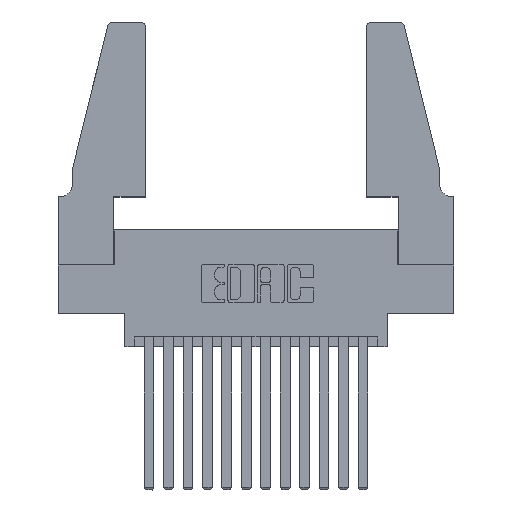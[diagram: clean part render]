
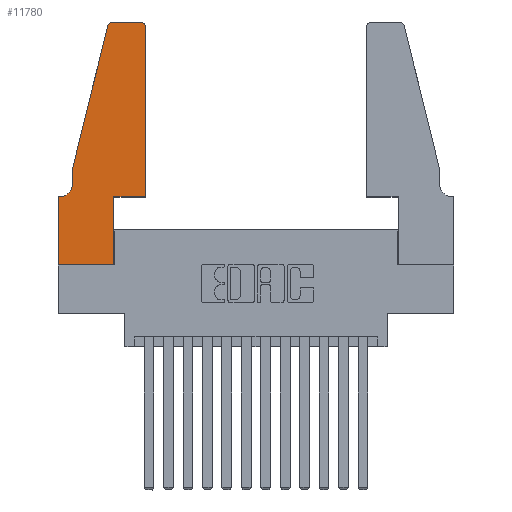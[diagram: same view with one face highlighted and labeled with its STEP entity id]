
A CAD part, top view. The second image highlights one B-rep face of the part: STEP entity #11780.
In plain terms, the highlighted planar face has unit normal (0, 0, 1).
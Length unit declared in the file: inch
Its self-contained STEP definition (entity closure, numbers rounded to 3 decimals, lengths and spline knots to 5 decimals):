
#50 = EDGE_CURVE ( 'NONE', #7303, #5042, #13932, .T. ) ;
#340 = DIRECTION ( 'NONE',  ( -0.239, -0.971, 0. ) ) ;
#411 = LINE ( 'NONE', #6189, #12069 ) ;
#577 = DIRECTION ( 'NONE',  ( 1., 0., 0. ) ) ;
#581 = CARTESIAN_POINT ( 'NONE',  ( 0., 0., 0.37 ) ) ;
#876 = CARTESIAN_POINT ( 'NONE',  ( 0.0055, 0.42, 0.37 ) ) ;
#1101 = CARTESIAN_POINT ( 'NONE',  ( 0.2865, 0., 0.37 ) ) ;
#1343 = ORIENTED_EDGE ( 'NONE', *, *, #13371, .T. ) ;
#1584 = CARTESIAN_POINT ( 'NONE',  ( 0.4205, 1.25, 0.37 ) ) ;
#1588 = DIRECTION ( 'NONE',  ( 0., 0., 1. ) ) ;
#1803 = CARTESIAN_POINT ( 'NONE',  ( 0.284, 1.22, 0.37 ) ) ;
#1908 = ORIENTED_EDGE ( 'NONE', *, *, #12167, .T. ) ;
#1970 = DIRECTION ( 'NONE',  ( 1., 0., 0. ) ) ;
#1988 = VERTEX_POINT ( 'NONE', #4067 ) ;
#2097 = VERTEX_POINT ( 'NONE', #13837 ) ;
#2110 = DIRECTION ( 'NONE',  ( 0., 0., -1. ) ) ;
#2118 = DIRECTION ( 'NONE',  ( 0., 1., 0. ) ) ;
#2516 = EDGE_CURVE ( 'NONE', #4257, #2097, #8026, .T. ) ;
#2548 = LINE ( 'NONE', #3177, #3809 ) ;
#2707 = VERTEX_POINT ( 'NONE', #11678 ) ;
#2776 = VECTOR ( 'NONE', #14270, 39.37008 ) ;
#2869 = VERTEX_POINT ( 'NONE', #1584 ) ;
#2880 = FACE_OUTER_BOUND ( 'NONE', #12619, .T. ) ;
#2902 = CARTESIAN_POINT ( 'NONE',  ( 0.4505, 0.35, 0.37 ) ) ;
#2933 = AXIS2_PLACEMENT_3D ( 'NONE', #1803, #6779, #1970 ) ;
#3019 = AXIS2_PLACEMENT_3D ( 'NONE', #876, #2110, #5719 ) ;
#3177 = CARTESIAN_POINT ( 'NONE',  ( 0.0755, 0.5, 0.37 ) ) ;
#3406 = VECTOR ( 'NONE', #7748, 39.37008 ) ;
#3809 = VECTOR ( 'NONE', #15198, 39.37008 ) ;
#4067 = CARTESIAN_POINT ( 'NONE',  ( 0.4505, 0.35, 0.37 ) ) ;
#4119 = LINE ( 'NONE', #10100, #3406 ) ;
#4257 = VERTEX_POINT ( 'NONE', #1101 ) ;
#5042 = VERTEX_POINT ( 'NONE', #15515 ) ;
#5075 = VERTEX_POINT ( 'NONE', #10425 ) ;
#5323 = CARTESIAN_POINT ( 'NONE',  ( 0.2605, 1.25, 0.37 ) ) ;
#5719 = DIRECTION ( 'NONE',  ( -1., 0., 0. ) ) ;
#5789 = VECTOR ( 'NONE', #11510, 39.37008 ) ;
#6189 = CARTESIAN_POINT ( 'NONE',  ( 0.0755, 0.35, 0.37 ) ) ;
#6210 = LINE ( 'NONE', #12662, #7722 ) ;
#6779 = DIRECTION ( 'NONE',  ( 0., 0., 1. ) ) ;
#7237 = EDGE_CURVE ( 'NONE', #13551, #9229, #15389, .T. ) ;
#7271 = CARTESIAN_POINT ( 'NONE',  ( 0.0755, 0.42, 0.37 ) ) ;
#7303 = VERTEX_POINT ( 'NONE', #12713 ) ;
#7722 = VECTOR ( 'NONE', #577, 39.37008 ) ;
#7748 = DIRECTION ( 'NONE',  ( 1., 0., 0. ) ) ;
#7757 = ORIENTED_EDGE ( 'NONE', *, *, #50, .T. ) ;
#8026 = LINE ( 'NONE', #11632, #2776 ) ;
#8221 = DIRECTION ( 'NONE',  ( 1., 0., 0. ) ) ;
#8367 = VECTOR ( 'NONE', #10159, 39.37008 ) ;
#8490 = ORIENTED_EDGE ( 'NONE', *, *, #10741, .T. ) ;
#8747 = DIRECTION ( 'NONE',  ( 1., 0., 0. ) ) ;
#8868 = CIRCLE ( 'NONE', #9159, 0.03 ) ;
#9159 = AXIS2_PLACEMENT_3D ( 'NONE', #10366, #12994, #8221 ) ;
#9229 = VERTEX_POINT ( 'NONE', #15496 ) ;
#9512 = LINE ( 'NONE', #5323, #8367 ) ;
#9833 = DIRECTION ( 'NONE',  ( -1., 0., 0. ) ) ;
#9992 = CARTESIAN_POINT ( 'NONE',  ( 0., 0.35, 0.37 ) ) ;
#10038 = AXIS2_PLACEMENT_3D ( 'NONE', #9992, #1588, #8747 ) ;
#10100 = CARTESIAN_POINT ( 'NONE',  ( 0., 0., 0.37 ) ) ;
#10159 = DIRECTION ( 'NONE',  ( -1., 0., 0. ) ) ;
#10269 = CARTESIAN_POINT ( 'NONE',  ( 0., 0.35, 0.37 ) ) ;
#10366 = CARTESIAN_POINT ( 'NONE',  ( 0.4205, 1.22, 0.37 ) ) ;
#10397 = LINE ( 'NONE', #12430, #13226 ) ;
#10425 = CARTESIAN_POINT ( 'NONE',  ( 0.0755, 0.5, 0.37 ) ) ;
#10494 = LINE ( 'NONE', #2902, #14815 ) ;
#10741 = EDGE_CURVE ( 'NONE', #2869, #7303, #9512, .T. ) ;
#11126 = ORIENTED_EDGE ( 'NONE', *, *, #11137, .T. ) ;
#11137 = EDGE_CURVE ( 'NONE', #5075, #11691, #2548, .T. ) ;
#11453 = EDGE_CURVE ( 'NONE', #2707, #13551, #411, .T. ) ;
#11500 = VERTEX_POINT ( 'NONE', #12369 ) ;
#11501 = EDGE_CURVE ( 'NONE', #5042, #5075, #10397, .T. ) ;
#11510 = DIRECTION ( 'NONE',  ( 0., -1., 0. ) ) ;
#11632 = CARTESIAN_POINT ( 'NONE',  ( 0.2865, 0.35, 0.37 ) ) ;
#11678 = CARTESIAN_POINT ( 'NONE',  ( 0.0055, 0.35, 0.37 ) ) ;
#11691 = VERTEX_POINT ( 'NONE', #7271 ) ;
#11780 = ADVANCED_FACE ( 'NONE', ( #2880 ), #12336, .T. ) ;
#11828 = ORIENTED_EDGE ( 'NONE', *, *, #13096, .T. ) ;
#12069 = VECTOR ( 'NONE', #9833, 39.37008 ) ;
#12167 = EDGE_CURVE ( 'NONE', #11691, #2707, #14682, .T. ) ;
#12336 = PLANE ( 'NONE',  #10038 ) ;
#12369 = CARTESIAN_POINT ( 'NONE',  ( 0.4505, 1.22, 0.37 ) ) ;
#12378 = ORIENTED_EDGE ( 'NONE', *, *, #2516, .T. ) ;
#12430 = CARTESIAN_POINT ( 'NONE',  ( 0.0755, 0.5, 0.37 ) ) ;
#12606 = EDGE_CURVE ( 'NONE', #11500, #2869, #8868, .T. ) ;
#12617 = ORIENTED_EDGE ( 'NONE', *, *, #11453, .T. ) ;
#12619 = EDGE_LOOP ( 'NONE', ( #8490, #7757, #14029, #11126, #1908, #12617, #13110, #1343, #12378, #11828, #13219, #13667 ) ) ;
#12662 = CARTESIAN_POINT ( 'NONE',  ( 0.4505, 0.35, 0.37 ) ) ;
#12713 = CARTESIAN_POINT ( 'NONE',  ( 0.284, 1.25, 0.37 ) ) ;
#12994 = DIRECTION ( 'NONE',  ( 0., 0., 1. ) ) ;
#13096 = EDGE_CURVE ( 'NONE', #2097, #1988, #6210, .T. ) ;
#13110 = ORIENTED_EDGE ( 'NONE', *, *, #7237, .T. ) ;
#13219 = ORIENTED_EDGE ( 'NONE', *, *, #14439, .T. ) ;
#13226 = VECTOR ( 'NONE', #340, 39.37008 ) ;
#13371 = EDGE_CURVE ( 'NONE', #9229, #4257, #4119, .T. ) ;
#13551 = VERTEX_POINT ( 'NONE', #10269 ) ;
#13667 = ORIENTED_EDGE ( 'NONE', *, *, #12606, .T. ) ;
#13837 = CARTESIAN_POINT ( 'NONE',  ( 0.2865, 0.35, 0.37 ) ) ;
#13932 = CIRCLE ( 'NONE', #2933, 0.03 ) ;
#14029 = ORIENTED_EDGE ( 'NONE', *, *, #11501, .T. ) ;
#14270 = DIRECTION ( 'NONE',  ( 0., 1., 0. ) ) ;
#14439 = EDGE_CURVE ( 'NONE', #1988, #11500, #10494, .T. ) ;
#14682 = CIRCLE ( 'NONE', #3019, 0.07 ) ;
#14815 = VECTOR ( 'NONE', #2118, 39.37008 ) ;
#15198 = DIRECTION ( 'NONE',  ( 0., -1., 0. ) ) ;
#15389 = LINE ( 'NONE', #581, #5789 ) ;
#15496 = CARTESIAN_POINT ( 'NONE',  ( 0., 0., 0.37 ) ) ;
#15515 = CARTESIAN_POINT ( 'NONE',  ( 0.25487, 1.22718, 0.37 ) ) ;
